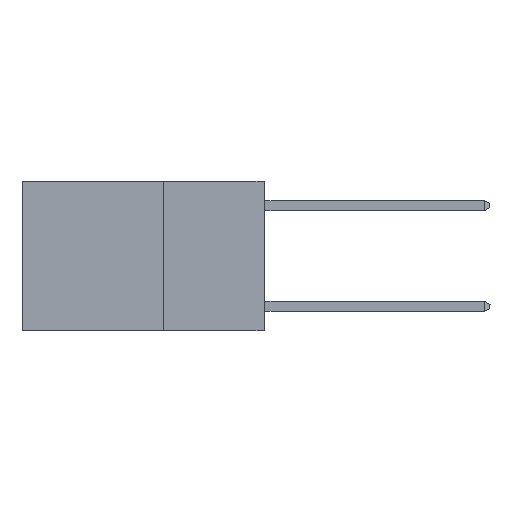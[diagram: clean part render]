
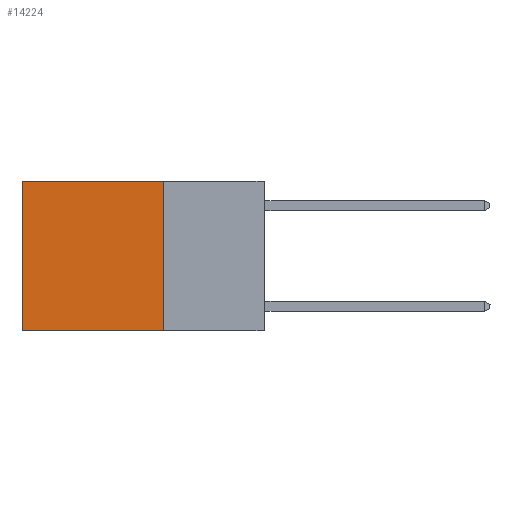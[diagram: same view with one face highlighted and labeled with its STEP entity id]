
A CAD part, left-side view. The second image highlights one B-rep face of the part: STEP entity #14224.
In plain terms, the highlighted planar face has unit normal (-1, 0, 0).
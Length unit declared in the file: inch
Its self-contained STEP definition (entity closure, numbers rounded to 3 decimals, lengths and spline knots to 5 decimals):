
#209 = ORIENTED_EDGE ( 'NONE', *, *, #2323, .F. ) ;
#585 = ORIENTED_EDGE ( 'NONE', *, *, #13714, .F. ) ;
#879 = ORIENTED_EDGE ( 'NONE', *, *, #17346, .T. ) ;
#943 = CARTESIAN_POINT ( 'NONE',  ( 0.2625, 0.25, 0. ) ) ;
#2323 = EDGE_CURVE ( 'NONE', #16303, #2571, #7162, .T. ) ;
#2571 = VERTEX_POINT ( 'NONE', #4561 ) ;
#3127 = VECTOR ( 'NONE', #6891, 39.37008 ) ;
#3647 = CARTESIAN_POINT ( 'NONE',  ( 0.2625, 0.25, -0.37 ) ) ;
#3934 = DIRECTION ( 'NONE',  ( 0., 0., -1. ) ) ;
#4122 = AXIS2_PLACEMENT_3D ( 'NONE', #943, #5689, #16441 ) ;
#4144 = PLANE ( 'NONE',  #4122 ) ;
#4561 = CARTESIAN_POINT ( 'NONE',  ( 0.2625, 0.6, -0.37 ) ) ;
#5250 = CARTESIAN_POINT ( 'NONE',  ( 0.2625, 0.25, 0. ) ) ;
#5689 = DIRECTION ( 'NONE',  ( 1., 0., 0. ) ) ;
#6891 = DIRECTION ( 'NONE',  ( 0., 1., 0. ) ) ;
#6980 = CARTESIAN_POINT ( 'NONE',  ( 0.2625, 0.6, 0. ) ) ;
#7162 = LINE ( 'NONE', #17608, #3127 ) ;
#9429 = ORIENTED_EDGE ( 'NONE', *, *, #17231, .T. ) ;
#9584 = CARTESIAN_POINT ( 'NONE',  ( 0.2625, 0.6, 0. ) ) ;
#10263 = VERTEX_POINT ( 'NONE', #5250 ) ;
#10412 = DIRECTION ( 'NONE',  ( 0., 0., -1. ) ) ;
#12039 = LINE ( 'NONE', #6980, #15681 ) ;
#13714 = EDGE_CURVE ( 'NONE', #10263, #16303, #19281, .T. ) ;
#13933 = FACE_OUTER_BOUND ( 'NONE', #15254, .T. ) ;
#14224 = ADVANCED_FACE ( 'NONE', ( #13933 ), #4144, .F. ) ;
#14253 = LINE ( 'NONE', #14956, #17755 ) ;
#14890 = DIRECTION ( 'NONE',  ( 0., 1., 0. ) ) ;
#14956 = CARTESIAN_POINT ( 'NONE',  ( 0.2625, 0.25, 0. ) ) ;
#15254 = EDGE_LOOP ( 'NONE', ( #9429, #209, #585, #879 ) ) ;
#15388 = VECTOR ( 'NONE', #10412, 39.37008 ) ;
#15681 = VECTOR ( 'NONE', #3934, 39.37008 ) ;
#16303 = VERTEX_POINT ( 'NONE', #3647 ) ;
#16441 = DIRECTION ( 'NONE',  ( 0., 0., -1. ) ) ;
#17231 = EDGE_CURVE ( 'NONE', #19303, #2571, #12039, .T. ) ;
#17346 = EDGE_CURVE ( 'NONE', #10263, #19303, #14253, .T. ) ;
#17608 = CARTESIAN_POINT ( 'NONE',  ( 0.2625, 0.25, -0.37 ) ) ;
#17755 = VECTOR ( 'NONE', #14890, 39.37008 ) ;
#18068 = CARTESIAN_POINT ( 'NONE',  ( 0.2625, 0.25, 0. ) ) ;
#19281 = LINE ( 'NONE', #18068, #15388 ) ;
#19303 = VERTEX_POINT ( 'NONE', #9584 ) ;
